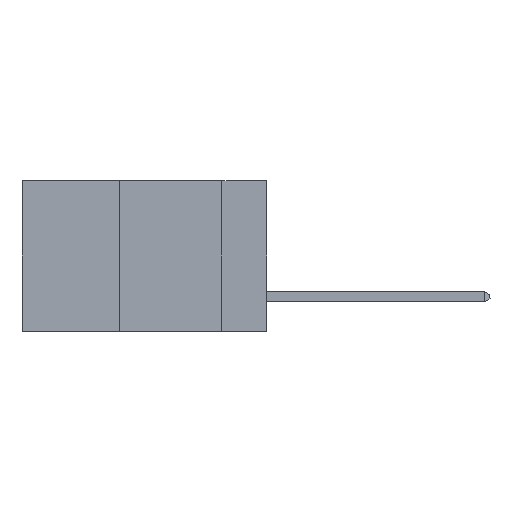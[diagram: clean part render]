
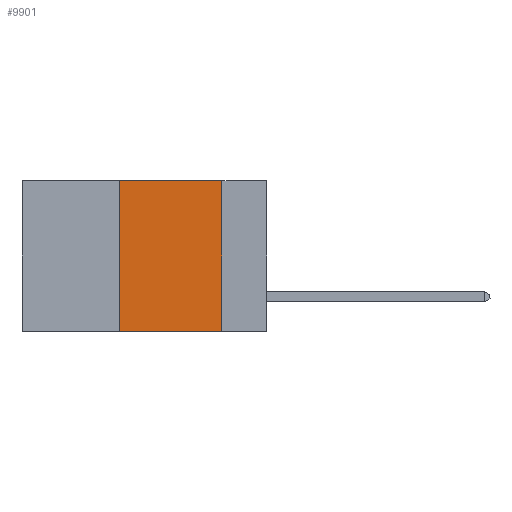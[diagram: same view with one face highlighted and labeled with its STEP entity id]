
A CAD part, left-side view. The second image highlights one B-rep face of the part: STEP entity #9901.
In plain terms, the highlighted planar face has unit normal (-1, 0, 0).
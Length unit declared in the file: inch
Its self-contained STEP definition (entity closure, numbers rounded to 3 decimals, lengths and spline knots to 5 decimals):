
#463 = EDGE_LOOP ( 'NONE', ( #13011, #26902, #2760, #23685 ) ) ;
#846 = VERTEX_POINT ( 'NONE', #13233 ) ;
#1205 = PLANE ( 'NONE',  #2474 ) ;
#1299 = VERTEX_POINT ( 'NONE', #12383 ) ;
#2474 = AXIS2_PLACEMENT_3D ( 'NONE', #15253, #17593, #3649 ) ;
#2760 = ORIENTED_EDGE ( 'NONE', *, *, #21886, .F. ) ;
#3649 = DIRECTION ( 'NONE',  ( 0., 0., -1. ) ) ;
#4006 = DIRECTION ( 'NONE',  ( 0., -1., 0. ) ) ;
#6544 = LINE ( 'NONE', #9225, #11304 ) ;
#6906 = VERTEX_POINT ( 'NONE', #30476 ) ;
#9225 = CARTESIAN_POINT ( 'NONE',  ( 0., 0.36, 0. ) ) ;
#9236 = VECTOR ( 'NONE', #17717, 39.37008 ) ;
#9901 = ADVANCED_FACE ( 'NONE', ( #21362 ), #1205, .F. ) ;
#10813 = LINE ( 'NONE', #11153, #16955 ) ;
#11153 = CARTESIAN_POINT ( 'NONE',  ( 0., 0.6, 0. ) ) ;
#11304 = VECTOR ( 'NONE', #23240, 39.37008 ) ;
#12383 = CARTESIAN_POINT ( 'NONE',  ( 0., 0.36, -0.37 ) ) ;
#13011 = ORIENTED_EDGE ( 'NONE', *, *, #28173, .F. ) ;
#13063 = CARTESIAN_POINT ( 'NONE',  ( 0., 0.6, -0.37 ) ) ;
#13233 = CARTESIAN_POINT ( 'NONE',  ( 0., 0.11, -0.37 ) ) ;
#13730 = DIRECTION ( 'NONE',  ( 0., 0., -1. ) ) ;
#15253 = CARTESIAN_POINT ( 'NONE',  ( 0., 0.6, 0. ) ) ;
#16955 = VECTOR ( 'NONE', #4006, 39.37008 ) ;
#17593 = DIRECTION ( 'NONE',  ( 1., 0., 0. ) ) ;
#17717 = DIRECTION ( 'NONE',  ( 0., -1., 0. ) ) ;
#20297 = EDGE_CURVE ( 'NONE', #1299, #846, #21629, .T. ) ;
#21185 = LINE ( 'NONE', #27737, #21949 ) ;
#21362 = FACE_OUTER_BOUND ( 'NONE', #463, .T. ) ;
#21629 = LINE ( 'NONE', #13063, #9236 ) ;
#21886 = EDGE_CURVE ( 'NONE', #1299, #6906, #6544, .T. ) ;
#21949 = VECTOR ( 'NONE', #13730, 39.37008 ) ;
#23240 = DIRECTION ( 'NONE',  ( 0., 0., 1. ) ) ;
#23267 = CARTESIAN_POINT ( 'NONE',  ( 0., 0.11, 0. ) ) ;
#23685 = ORIENTED_EDGE ( 'NONE', *, *, #20297, .T. ) ;
#23688 = EDGE_CURVE ( 'NONE', #6906, #28245, #10813, .T. ) ;
#26902 = ORIENTED_EDGE ( 'NONE', *, *, #23688, .F. ) ;
#27737 = CARTESIAN_POINT ( 'NONE',  ( 0., 0.11, 0. ) ) ;
#28173 = EDGE_CURVE ( 'NONE', #28245, #846, #21185, .T. ) ;
#28245 = VERTEX_POINT ( 'NONE', #23267 ) ;
#30476 = CARTESIAN_POINT ( 'NONE',  ( 0., 0.36, 0. ) ) ;
